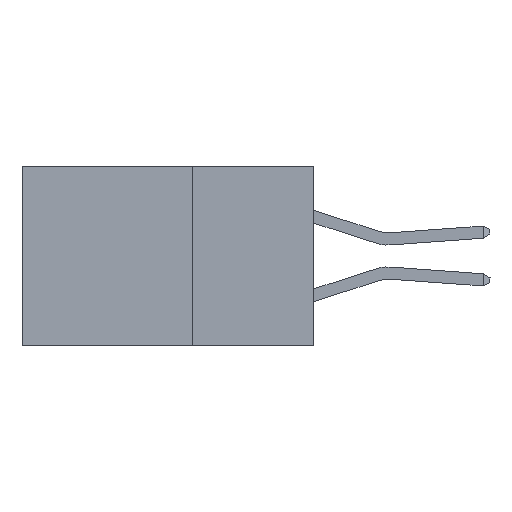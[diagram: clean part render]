
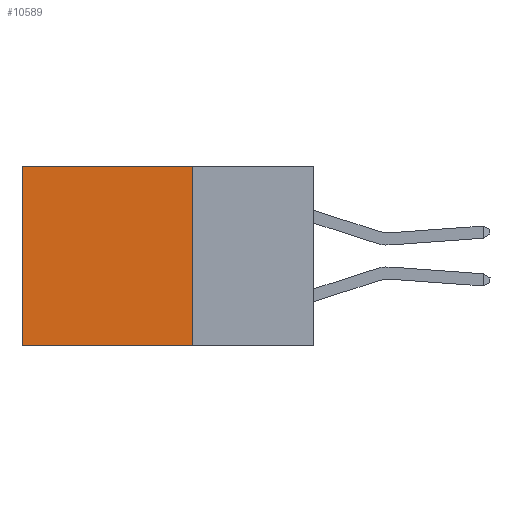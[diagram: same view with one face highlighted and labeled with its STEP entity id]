
A CAD part, left-side view. The second image highlights one B-rep face of the part: STEP entity #10589.
In plain terms, the highlighted planar face has unit normal (-1, 0, 0).
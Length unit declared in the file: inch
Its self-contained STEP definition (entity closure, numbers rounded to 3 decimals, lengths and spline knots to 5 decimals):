
#423 = ORIENTED_EDGE ( 'NONE', *, *, #23644, .T. ) ;
#1227 = CARTESIAN_POINT ( 'NONE',  ( 0.2875, 0.25, 0. ) ) ;
#1514 = DIRECTION ( 'NONE',  ( 0., 0., -1. ) ) ;
#1604 = DIRECTION ( 'NONE',  ( 0., 0., -1. ) ) ;
#2134 = DIRECTION ( 'NONE',  ( 1., 0., 0. ) ) ;
#3400 = EDGE_CURVE ( 'NONE', #4142, #10107, #23905, .T. ) ;
#3437 = CARTESIAN_POINT ( 'NONE',  ( 0.2875, 0.6, -0.37 ) ) ;
#4142 = VERTEX_POINT ( 'NONE', #10499 ) ;
#4863 = EDGE_CURVE ( 'NONE', #4142, #10806, #12335, .T. ) ;
#5505 = VERTEX_POINT ( 'NONE', #3437 ) ;
#6973 = ORIENTED_EDGE ( 'NONE', *, *, #4863, .T. ) ;
#7436 = VECTOR ( 'NONE', #16712, 39.37008 ) ;
#7951 = EDGE_LOOP ( 'NONE', ( #423, #12400, #13022, #6973 ) ) ;
#10107 = VERTEX_POINT ( 'NONE', #12023 ) ;
#10499 = CARTESIAN_POINT ( 'NONE',  ( 0.2875, 0.25, 0. ) ) ;
#10589 = ADVANCED_FACE ( 'NONE', ( #20183 ), #13301, .F. ) ;
#10787 = DIRECTION ( 'NONE',  ( 0., 1., 0. ) ) ;
#10806 = VERTEX_POINT ( 'NONE', #17500 ) ;
#10949 = CARTESIAN_POINT ( 'NONE',  ( 0.2875, 0.6, 0. ) ) ;
#11455 = CARTESIAN_POINT ( 'NONE',  ( 0.2875, 0.25, 0. ) ) ;
#12023 = CARTESIAN_POINT ( 'NONE',  ( 0.2875, 0.25, -0.37 ) ) ;
#12335 = LINE ( 'NONE', #16816, #7436 ) ;
#12400 = ORIENTED_EDGE ( 'NONE', *, *, #21751, .F. ) ;
#12413 = VECTOR ( 'NONE', #1604, 39.37008 ) ;
#12993 = LINE ( 'NONE', #10949, #12413 ) ;
#13022 = ORIENTED_EDGE ( 'NONE', *, *, #3400, .F. ) ;
#13301 = PLANE ( 'NONE',  #15655 ) ;
#14729 = VECTOR ( 'NONE', #1514, 39.37008 ) ;
#15149 = DIRECTION ( 'NONE',  ( 0., 0., -1. ) ) ;
#15655 = AXIS2_PLACEMENT_3D ( 'NONE', #11455, #2134, #15149 ) ;
#16712 = DIRECTION ( 'NONE',  ( 0., 1., 0. ) ) ;
#16816 = CARTESIAN_POINT ( 'NONE',  ( 0.2875, 0.25, 0. ) ) ;
#17380 = VECTOR ( 'NONE', #10787, 39.37008 ) ;
#17500 = CARTESIAN_POINT ( 'NONE',  ( 0.2875, 0.6, 0. ) ) ;
#17956 = LINE ( 'NONE', #19926, #17380 ) ;
#19926 = CARTESIAN_POINT ( 'NONE',  ( 0.2875, 0.25, -0.37 ) ) ;
#20183 = FACE_OUTER_BOUND ( 'NONE', #7951, .T. ) ;
#21751 = EDGE_CURVE ( 'NONE', #10107, #5505, #17956, .T. ) ;
#23644 = EDGE_CURVE ( 'NONE', #10806, #5505, #12993, .T. ) ;
#23905 = LINE ( 'NONE', #1227, #14729 ) ;
